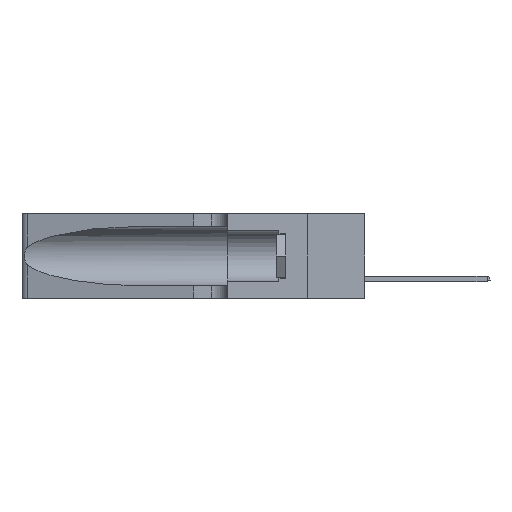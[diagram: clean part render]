
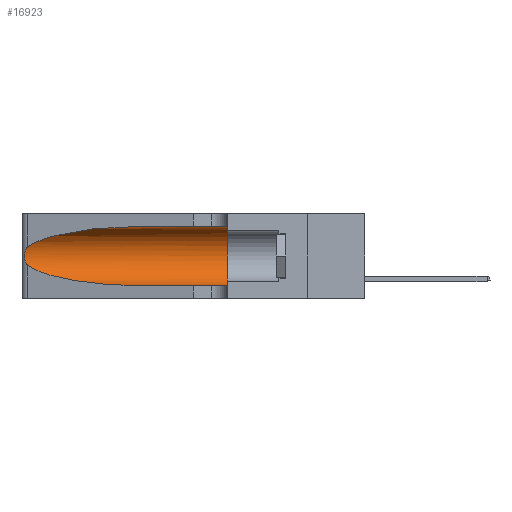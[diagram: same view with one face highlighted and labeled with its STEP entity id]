
A CAD part, left-side view. The second image highlights one B-rep face of the part: STEP entity #16923.
In plain terms, the highlighted cylindrical face has radius 3.308 mm (diameter 6.617 mm), a partial arc.
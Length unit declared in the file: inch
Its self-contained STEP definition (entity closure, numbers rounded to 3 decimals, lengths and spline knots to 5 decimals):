
#8 = EDGE_CURVE ( 'NONE', #11350, #14625, #7925, .T. ) ;
#365 = CARTESIAN_POINT ( 'NONE',  ( 0.2373, 1.15595, 0.08982 ) ) ;
#830 = CARTESIAN_POINT ( 'NONE',  ( 0.1305, 0.72297, 0.05475 ) ) ;
#835 = ORIENTED_EDGE ( 'NONE', *, *, #8, .T. ) ;
#1114 = CARTESIAN_POINT ( 'NONE',  ( 0.25487, 1.22718, 0.14631 ) ) ;
#1422 =( BOUNDED_CURVE ( )  B_SPLINE_CURVE ( 3, ( #4705, #8481, #3104, #21742 ),
 .UNSPECIFIED., .F., .T. ) 
 B_SPLINE_CURVE_WITH_KNOTS ( ( 4, 4 ),
 ( 1.5708, 2.84003 ),
 .UNSPECIFIED. ) 
 CURVE ( )  GEOMETRIC_REPRESENTATION_ITEM ( )  RATIONAL_B_SPLINE_CURVE ( ( 1., 0.87, 0.87, 1. ) ) 
 REPRESENTATION_ITEM ( '' )  );
#1973 = VERTEX_POINT ( 'NONE', #12320 ) ;
#2090 = CARTESIAN_POINT ( 'NONE',  ( 0.18966, 0.96281, 0.05475 ) ) ;
#2532 = EDGE_CURVE ( 'NONE', #11311, #11350, #7611, .T. ) ;
#2781 = CARTESIAN_POINT ( 'NONE',  ( 0.25555, 1.22994, 0.2215 ) ) ;
#2838 = EDGE_CURVE ( 'NONE', #10350, #1973, #14996, .T. ) ;
#2862 = CARTESIAN_POINT ( 'NONE',  ( 0.25856, 1.23593, 0.16098 ) ) ;
#2872 = CARTESIAN_POINT ( 'NONE',  ( 0.1305, 0.72297, 0.31525 ) ) ;
#2965 = AXIS2_PLACEMENT_3D ( 'NONE', #14414, #24184, #5070 ) ;
#3034 = CARTESIAN_POINT ( 'NONE',  ( 0.25487, 1.22718, 0.22369 ) ) ;
#3104 = CARTESIAN_POINT ( 'NONE',  ( 0.2373, 1.15595, 0.28018 ) ) ;
#3533 = ORIENTED_EDGE ( 'NONE', *, *, #2532, .T. ) ;
#4705 = CARTESIAN_POINT ( 'NONE',  ( 0.1305, 0.72297, 0.31525 ) ) ;
#4793 = ORIENTED_EDGE ( 'NONE', *, *, #14430, .F. ) ;
#5070 = DIRECTION ( 'NONE',  ( 0., 0., -1. ) ) ;
#5331 = DIRECTION ( 'NONE',  ( 0., 0., 1. ) ) ;
#6290 = CARTESIAN_POINT ( 'NONE',  ( 0.25487, 1.22718, 0.22369 ) ) ;
#7023 = DIRECTION ( 'NONE',  ( 0., -1., 0. ) ) ;
#7611 = B_SPLINE_CURVE_WITH_KNOTS ( 'NONE', 3,
 ( #3034, #2781, #8805, #21835, #16022, #19838, #23900, #17926, #8723, #2862, #10479, #23657, #12294, #1114 ),
 .UNSPECIFIED., .F., .F.,
 ( 4, 2, 2, 2, 2, 2, 4 ),
 ( 0., 0.00027, 0.00053, 0.00107, 0.0016, 0.00187, 0.00214 ),
 .UNSPECIFIED. ) ;
#7925 =( BOUNDED_CURVE ( )  B_SPLINE_CURVE ( 3, ( #9785, #365, #2090, #13611 ),
 .UNSPECIFIED., .F., .T. ) 
 B_SPLINE_CURVE_WITH_KNOTS ( ( 4, 4 ),
 ( 3.44316, 4.71239 ),
 .UNSPECIFIED. ) 
 CURVE ( )  GEOMETRIC_REPRESENTATION_ITEM ( )  RATIONAL_B_SPLINE_CURVE ( ( 1., 0.87, 0.87, 1. ) ) 
 REPRESENTATION_ITEM ( '' )  );
#8481 = CARTESIAN_POINT ( 'NONE',  ( 0.18966, 0.96281, 0.31525 ) ) ;
#8610 = ORIENTED_EDGE ( 'NONE', *, *, #2838, .F. ) ;
#8723 = CARTESIAN_POINT ( 'NONE',  ( 0.26017, 1.23833, 0.17102 ) ) ;
#8805 = CARTESIAN_POINT ( 'NONE',  ( 0.25639, 1.23184, 0.21858 ) ) ;
#9667 = LINE ( 'NONE', #23936, #14409 ) ;
#9785 = CARTESIAN_POINT ( 'NONE',  ( 0.25487, 1.22718, 0.14631 ) ) ;
#10027 = FACE_OUTER_BOUND ( 'NONE', #24446, .T. ) ;
#10038 = EDGE_CURVE ( 'NONE', #18593, #11311, #1422, .T. ) ;
#10350 = VERTEX_POINT ( 'NONE', #11951 ) ;
#10479 = CARTESIAN_POINT ( 'NONE',  ( 0.25789, 1.23486, 0.15765 ) ) ;
#10530 = LINE ( 'NONE', #17985, #19094 ) ;
#11109 = CARTESIAN_POINT ( 'NONE',  ( 0.1305, 0.35, 0.185 ) ) ;
#11311 = VERTEX_POINT ( 'NONE', #6290 ) ;
#11350 = VERTEX_POINT ( 'NONE', #17873 ) ;
#11951 = CARTESIAN_POINT ( 'NONE',  ( 0.1305, 0.35, 0.31525 ) ) ;
#12294 = CARTESIAN_POINT ( 'NONE',  ( 0.25555, 1.22993, 0.14849 ) ) ;
#12320 = CARTESIAN_POINT ( 'NONE',  ( 0.1305, 0.35, 0.05475 ) ) ;
#12853 = DIRECTION ( 'NONE',  ( 0., 1., 0. ) ) ;
#13611 = CARTESIAN_POINT ( 'NONE',  ( 0.1305, 0.72297, 0.05475 ) ) ;
#13959 = ORIENTED_EDGE ( 'NONE', *, *, #10038, .T. ) ;
#14409 = VECTOR ( 'NONE', #7023, 39.37008 ) ;
#14414 = CARTESIAN_POINT ( 'NONE',  ( 0.1305, 1.61858, 0.185 ) ) ;
#14430 = EDGE_CURVE ( 'NONE', #18593, #10350, #9667, .T. ) ;
#14625 = VERTEX_POINT ( 'NONE', #830 ) ;
#14996 = CIRCLE ( 'NONE', #17967, 0.13025 ) ;
#16022 = CARTESIAN_POINT ( 'NONE',  ( 0.25854, 1.2359, 0.20912 ) ) ;
#16844 = ORIENTED_EDGE ( 'NONE', *, *, #19125, .T. ) ;
#16923 = ADVANCED_FACE ( 'NONE', ( #10027 ), #22753, .F. ) ;
#17873 = CARTESIAN_POINT ( 'NONE',  ( 0.25487, 1.22718, 0.14631 ) ) ;
#17926 = CARTESIAN_POINT ( 'NONE',  ( 0.26075, 1.23896, 0.178 ) ) ;
#17967 = AXIS2_PLACEMENT_3D ( 'NONE', #11109, #12853, #5331 ) ;
#17985 = CARTESIAN_POINT ( 'NONE',  ( 0.1305, 1.61858, 0.05475 ) ) ;
#18593 = VERTEX_POINT ( 'NONE', #2872 ) ;
#19094 = VECTOR ( 'NONE', #19896, 39.37008 ) ;
#19125 = EDGE_CURVE ( 'NONE', #14625, #1973, #10530, .T. ) ;
#19838 = CARTESIAN_POINT ( 'NONE',  ( 0.26018, 1.23835, 0.19895 ) ) ;
#19896 = DIRECTION ( 'NONE',  ( 0., -1., 0. ) ) ;
#21742 = CARTESIAN_POINT ( 'NONE',  ( 0.25487, 1.22718, 0.22369 ) ) ;
#21835 = CARTESIAN_POINT ( 'NONE',  ( 0.25787, 1.23484, 0.2124 ) ) ;
#22753 = CYLINDRICAL_SURFACE ( 'NONE', #2965, 0.13025 ) ;
#23657 = CARTESIAN_POINT ( 'NONE',  ( 0.25639, 1.23186, 0.15144 ) ) ;
#23900 = CARTESIAN_POINT ( 'NONE',  ( 0.26075, 1.23896, 0.19203 ) ) ;
#23936 = CARTESIAN_POINT ( 'NONE',  ( 0.1305, 1.61858, 0.31525 ) ) ;
#24184 = DIRECTION ( 'NONE',  ( 0., -1., 0. ) ) ;
#24446 = EDGE_LOOP ( 'NONE', ( #13959, #3533, #835, #16844, #8610, #4793 ) ) ;
